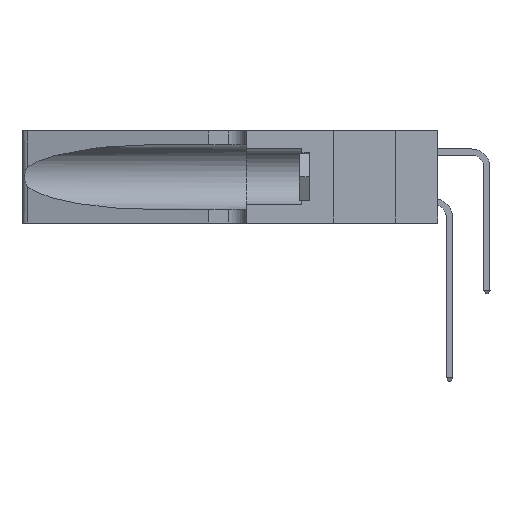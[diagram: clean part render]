
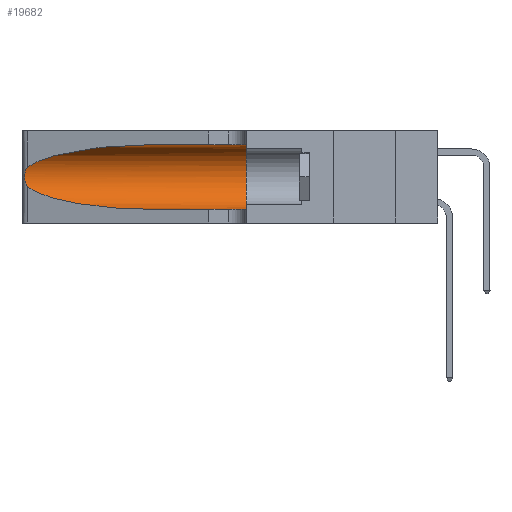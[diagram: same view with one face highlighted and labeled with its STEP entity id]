
A CAD part, left-side view. The second image highlights one B-rep face of the part: STEP entity #19682.
In plain terms, the highlighted cylindrical face has radius 3.308 mm (diameter 6.617 mm), a partial arc.
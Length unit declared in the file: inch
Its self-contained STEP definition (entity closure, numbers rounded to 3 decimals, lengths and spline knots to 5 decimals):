
#422 = CARTESIAN_POINT ( 'NONE',  ( 0.25487, 1.22718, 0.22369 ) ) ;
#1875 = VERTEX_POINT ( 'NONE', #4715 ) ;
#2219 = ORIENTED_EDGE ( 'NONE', *, *, #27172, .F. ) ;
#3249 = DIRECTION ( 'NONE',  ( 0., 1., 0. ) ) ;
#3426 = CARTESIAN_POINT ( 'NONE',  ( 0.25555, 1.22994, 0.2215 ) ) ;
#3523 = CARTESIAN_POINT ( 'NONE',  ( 0.25487, 1.22718, 0.14631 ) ) ;
#3852 = ORIENTED_EDGE ( 'NONE', *, *, #6216, .F. ) ;
#4070 = ORIENTED_EDGE ( 'NONE', *, *, #13682, .T. ) ;
#4200 = VECTOR ( 'NONE', #26807, 39.37008 ) ;
#4693 = ORIENTED_EDGE ( 'NONE', *, *, #5286, .T. ) ;
#4715 = CARTESIAN_POINT ( 'NONE',  ( 0.1305, 0.35, 0.05475 ) ) ;
#5286 = EDGE_CURVE ( 'NONE', #9907, #1875, #22237, .T. ) ;
#5654 = CARTESIAN_POINT ( 'NONE',  ( 0.26017, 1.23833, 0.17102 ) ) ;
#5762 = CARTESIAN_POINT ( 'NONE',  ( 0.26075, 1.23896, 0.19203 ) ) ;
#5928 = CARTESIAN_POINT ( 'NONE',  ( 0.1305, 1.61858, 0.05475 ) ) ;
#6216 = EDGE_CURVE ( 'NONE', #28566, #29211, #11922, .T. ) ;
#7650 =( BOUNDED_CURVE ( )  B_SPLINE_CURVE ( 3, ( #9612, #23739, #14502, #17164 ),
 .UNSPECIFIED., .F., .F. ) 
 B_SPLINE_CURVE_WITH_KNOTS ( ( 4, 4 ),
 ( 3.44316, 4.71239 ),
 .UNSPECIFIED. ) 
 CURVE ( )  GEOMETRIC_REPRESENTATION_ITEM ( )  RATIONAL_B_SPLINE_CURVE ( ( 1., 0.87, 0.87, 1. ) ) 
 REPRESENTATION_ITEM ( '' )  );
#7972 = DIRECTION ( 'NONE',  ( 0., 0., 1. ) ) ;
#8134 = CARTESIAN_POINT ( 'NONE',  ( 0.26075, 1.23896, 0.178 ) ) ;
#8669 = ORIENTED_EDGE ( 'NONE', *, *, #13872, .T. ) ;
#8732 = ORIENTED_EDGE ( 'NONE', *, *, #29425, .T. ) ;
#9399 = VERTEX_POINT ( 'NONE', #21456 ) ;
#9612 = CARTESIAN_POINT ( 'NONE',  ( 0.25487, 1.22718, 0.14631 ) ) ;
#9907 = VERTEX_POINT ( 'NONE', #24864 ) ;
#10051 = AXIS2_PLACEMENT_3D ( 'NONE', #12415, #21603, #14843 ) ;
#10433 = VERTEX_POINT ( 'NONE', #20609 ) ;
#10502 = CARTESIAN_POINT ( 'NONE',  ( 0.25487, 1.22718, 0.22369 ) ) ;
#10612 = CARTESIAN_POINT ( 'NONE',  ( 0.1305, 1.61858, 0.31525 ) ) ;
#11922 = LINE ( 'NONE', #10612, #4200 ) ;
#12088 = FACE_OUTER_BOUND ( 'NONE', #21314, .T. ) ;
#12415 = CARTESIAN_POINT ( 'NONE',  ( 0.1305, 1.61858, 0.185 ) ) ;
#12610 = CARTESIAN_POINT ( 'NONE',  ( 0.1305, 0.35, 0.185 ) ) ;
#12884 = CARTESIAN_POINT ( 'NONE',  ( 0.25639, 1.23186, 0.15144 ) ) ;
#13682 = EDGE_CURVE ( 'NONE', #28566, #9399, #29316, .T. ) ;
#13872 = EDGE_CURVE ( 'NONE', #9399, #10433, #23837, .T. ) ;
#14502 = CARTESIAN_POINT ( 'NONE',  ( 0.18966, 0.96281, 0.05475 ) ) ;
#14843 = DIRECTION ( 'NONE',  ( 0., 0., -1. ) ) ;
#15017 = CARTESIAN_POINT ( 'NONE',  ( 0.25787, 1.23484, 0.2124 ) ) ;
#15829 = CARTESIAN_POINT ( 'NONE',  ( 0.1305, 0.72297, 0.31525 ) ) ;
#15898 = CARTESIAN_POINT ( 'NONE',  ( 0.1305, 0.35, 0.31525 ) ) ;
#16758 = CARTESIAN_POINT ( 'NONE',  ( 0.2373, 1.15595, 0.28018 ) ) ;
#17144 = CARTESIAN_POINT ( 'NONE',  ( 0.18966, 0.96281, 0.31525 ) ) ;
#17164 = CARTESIAN_POINT ( 'NONE',  ( 0.1305, 0.72297, 0.05475 ) ) ;
#19682 = ADVANCED_FACE ( 'NONE', ( #12088 ), #27098, .F. ) ;
#19696 = CARTESIAN_POINT ( 'NONE',  ( 0.25854, 1.2359, 0.20912 ) ) ;
#19803 = CARTESIAN_POINT ( 'NONE',  ( 0.25639, 1.23184, 0.21858 ) ) ;
#20609 = CARTESIAN_POINT ( 'NONE',  ( 0.25487, 1.22718, 0.14631 ) ) ;
#20966 = AXIS2_PLACEMENT_3D ( 'NONE', #12610, #3249, #7972 ) ;
#21314 = EDGE_LOOP ( 'NONE', ( #4070, #8669, #8732, #4693, #2219, #3852 ) ) ;
#21456 = CARTESIAN_POINT ( 'NONE',  ( 0.25487, 1.22718, 0.22369 ) ) ;
#21603 = DIRECTION ( 'NONE',  ( 0., -1., 0. ) ) ;
#22237 = LINE ( 'NONE', #5928, #26267 ) ;
#23739 = CARTESIAN_POINT ( 'NONE',  ( 0.2373, 1.15595, 0.08982 ) ) ;
#23837 = B_SPLINE_CURVE_WITH_KNOTS ( 'NONE', 3,
 ( #10502, #3426, #19803, #15017, #19696, #24635, #5762, #8134, #5654, #27100, #26897, #12884, #29266, #3523 ),
 .UNSPECIFIED., .F., .F.,
 ( 4, 2, 2, 2, 2, 2, 4 ),
 ( 0., 0.00027, 0.00053, 0.00107, 0.0016, 0.00187, 0.00214 ),
 .UNSPECIFIED. ) ;
#24111 = CARTESIAN_POINT ( 'NONE',  ( 0.1305, 0.72297, 0.31525 ) ) ;
#24635 = CARTESIAN_POINT ( 'NONE',  ( 0.26018, 1.23835, 0.19895 ) ) ;
#24702 = DIRECTION ( 'NONE',  ( 0., -1., 0. ) ) ;
#24864 = CARTESIAN_POINT ( 'NONE',  ( 0.1305, 0.72297, 0.05475 ) ) ;
#26267 = VECTOR ( 'NONE', #24702, 39.37008 ) ;
#26321 = CIRCLE ( 'NONE', #20966, 0.13025 ) ;
#26807 = DIRECTION ( 'NONE',  ( 0., -1., 0. ) ) ;
#26897 = CARTESIAN_POINT ( 'NONE',  ( 0.25789, 1.23486, 0.15765 ) ) ;
#27098 = CYLINDRICAL_SURFACE ( 'NONE', #10051, 0.13025 ) ;
#27100 = CARTESIAN_POINT ( 'NONE',  ( 0.25856, 1.23593, 0.16098 ) ) ;
#27172 = EDGE_CURVE ( 'NONE', #29211, #1875, #26321, .T. ) ;
#28566 = VERTEX_POINT ( 'NONE', #15829 ) ;
#29211 = VERTEX_POINT ( 'NONE', #15898 ) ;
#29266 = CARTESIAN_POINT ( 'NONE',  ( 0.25555, 1.22993, 0.14849 ) ) ;
#29316 =( BOUNDED_CURVE ( )  B_SPLINE_CURVE ( 3, ( #24111, #17144, #16758, #422 ),
 .UNSPECIFIED., .F., .F. ) 
 B_SPLINE_CURVE_WITH_KNOTS ( ( 4, 4 ),
 ( 1.5708, 2.84003 ),
 .UNSPECIFIED. ) 
 CURVE ( )  GEOMETRIC_REPRESENTATION_ITEM ( )  RATIONAL_B_SPLINE_CURVE ( ( 1., 0.87, 0.87, 1. ) ) 
 REPRESENTATION_ITEM ( '' )  );
#29425 = EDGE_CURVE ( 'NONE', #10433, #9907, #7650, .T. ) ;
